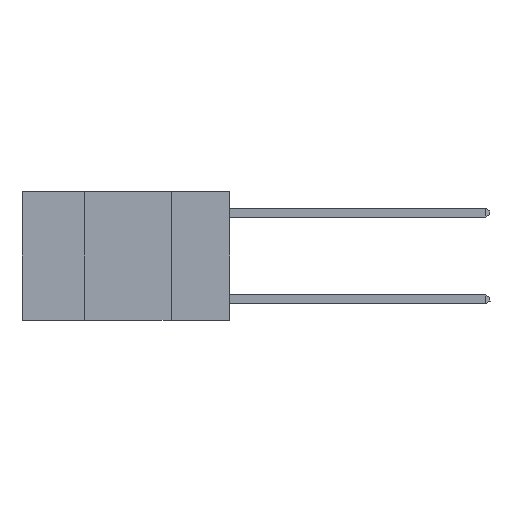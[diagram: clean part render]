
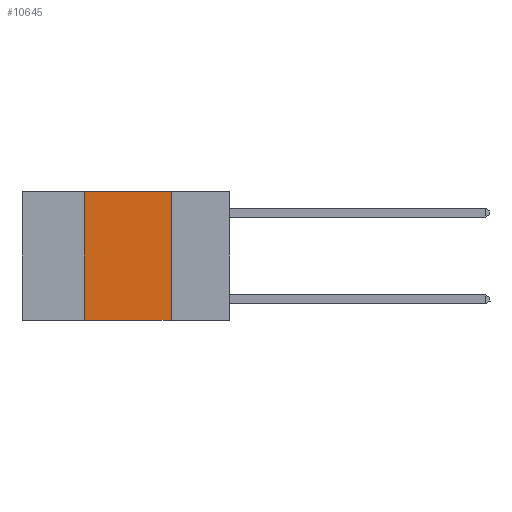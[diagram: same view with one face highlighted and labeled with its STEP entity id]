
A CAD part, left-side view. The second image highlights one B-rep face of the part: STEP entity #10645.
In plain terms, the highlighted planar face has unit normal (-1, 0, 0).
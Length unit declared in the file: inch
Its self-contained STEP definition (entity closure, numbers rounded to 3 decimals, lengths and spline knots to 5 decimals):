
#1088 = LINE ( 'NONE', #6681, #5290 ) ;
#1451 = CARTESIAN_POINT ( 'NONE',  ( 0., 0.17, 0. ) ) ;
#2529 = VECTOR ( 'NONE', #10231, 39.37008 ) ;
#3015 = PLANE ( 'NONE',  #15885 ) ;
#3096 = LINE ( 'NONE', #1451, #2529 ) ;
#3200 = VECTOR ( 'NONE', #5620, 39.37008 ) ;
#3482 = ORIENTED_EDGE ( 'NONE', *, *, #13935, .F. ) ;
#4028 = ORIENTED_EDGE ( 'NONE', *, *, #10416, .T. ) ;
#4354 = FACE_OUTER_BOUND ( 'NONE', #11367, .T. ) ;
#4797 = CARTESIAN_POINT ( 'NONE',  ( 0., 0.6, 0. ) ) ;
#5290 = VECTOR ( 'NONE', #11850, 39.37008 ) ;
#5620 = DIRECTION ( 'NONE',  ( 0., 0., 1. ) ) ;
#6620 = DIRECTION ( 'NONE',  ( 1., 0., 0. ) ) ;
#6681 = CARTESIAN_POINT ( 'NONE',  ( 0., 0.6, 0. ) ) ;
#8221 = VECTOR ( 'NONE', #21077, 39.37008 ) ;
#8243 = EDGE_CURVE ( 'NONE', #14034, #21332, #1088, .T. ) ;
#9794 = VERTEX_POINT ( 'NONE', #10548 ) ;
#10231 = DIRECTION ( 'NONE',  ( 0., 0., -1. ) ) ;
#10416 = EDGE_CURVE ( 'NONE', #9794, #10864, #17475, .T. ) ;
#10528 = CARTESIAN_POINT ( 'NONE',  ( 0., 0.6, -0.37 ) ) ;
#10548 = CARTESIAN_POINT ( 'NONE',  ( 0., 0.42, -0.37 ) ) ;
#10645 = ADVANCED_FACE ( 'NONE', ( #4354 ), #3015, .F. ) ;
#10864 = VERTEX_POINT ( 'NONE', #14127 ) ;
#11367 = EDGE_LOOP ( 'NONE', ( #3482, #17422, #21944, #4028 ) ) ;
#11610 = EDGE_CURVE ( 'NONE', #9794, #14034, #21119, .T. ) ;
#11850 = DIRECTION ( 'NONE',  ( 0., -1., 0. ) ) ;
#12939 = CARTESIAN_POINT ( 'NONE',  ( 0., 0.17, 0. ) ) ;
#13935 = EDGE_CURVE ( 'NONE', #21332, #10864, #3096, .T. ) ;
#14034 = VERTEX_POINT ( 'NONE', #17445 ) ;
#14127 = CARTESIAN_POINT ( 'NONE',  ( 0., 0.17, -0.37 ) ) ;
#15885 = AXIS2_PLACEMENT_3D ( 'NONE', #4797, #6620, #18719 ) ;
#17422 = ORIENTED_EDGE ( 'NONE', *, *, #8243, .F. ) ;
#17445 = CARTESIAN_POINT ( 'NONE',  ( 0., 0.42, 0. ) ) ;
#17475 = LINE ( 'NONE', #10528, #8221 ) ;
#17787 = CARTESIAN_POINT ( 'NONE',  ( 0., 0.42, 0. ) ) ;
#18719 = DIRECTION ( 'NONE',  ( 0., 0., -1. ) ) ;
#21077 = DIRECTION ( 'NONE',  ( 0., -1., 0. ) ) ;
#21119 = LINE ( 'NONE', #17787, #3200 ) ;
#21332 = VERTEX_POINT ( 'NONE', #12939 ) ;
#21944 = ORIENTED_EDGE ( 'NONE', *, *, #11610, .F. ) ;
